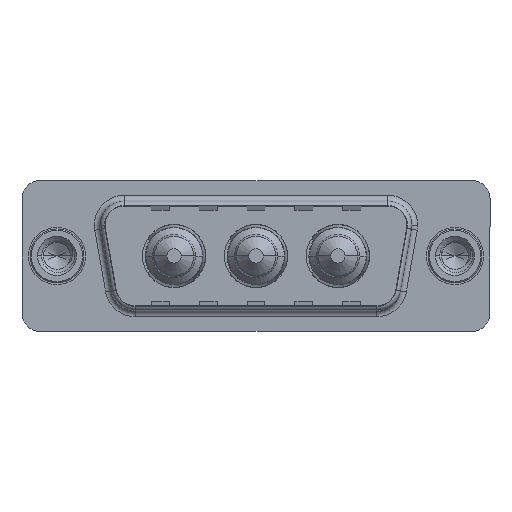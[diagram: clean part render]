
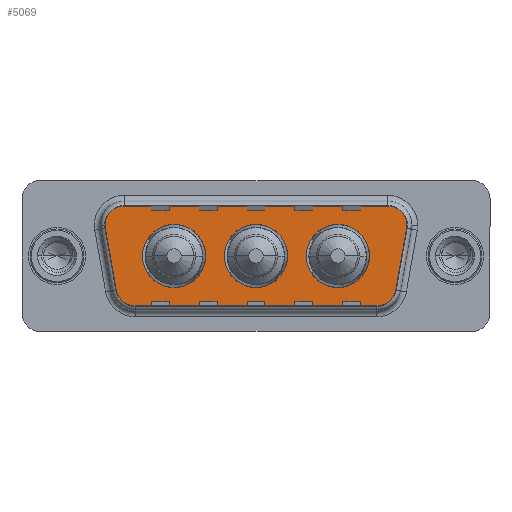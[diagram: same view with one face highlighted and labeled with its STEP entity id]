
A CAD part, top view. The second image highlights one B-rep face of the part: STEP entity #5069.
In plain terms, the highlighted planar face has unit normal (0, 0, 1).
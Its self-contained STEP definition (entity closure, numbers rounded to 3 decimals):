
#84 = VECTOR ( 'NONE', #6820, 1000. ) ;
#132 = EDGE_CURVE ( 'NONE', #2947, #4873, #10648, .T. ) ;
#138 = AXIS2_PLACEMENT_3D ( 'NONE', #4179, #12192, #12235 ) ;
#210 = FACE_OUTER_BOUND ( 'NONE', #10993, .T. ) ;
#246 = CIRCLE ( 'NONE', #1196, 2.65 ) ;
#299 = LINE ( 'NONE', #9183, #2934 ) ;
#313 = EDGE_CURVE ( 'NONE', #2612, #9984, #11903, .T. ) ;
#733 = CARTESIAN_POINT ( 'NONE',  ( 9.8, 0., 0. ) ) ;
#816 = CARTESIAN_POINT ( 'NONE',  ( 19.3, 0., 0. ) ) ;
#866 = ORIENTED_EDGE ( 'NONE', *, *, #8293, .T. ) ;
#870 = VERTEX_POINT ( 'NONE', #6305 ) ;
#885 = CARTESIAN_POINT ( 'NONE',  ( 4.464, -3.247, 0. ) ) ;
#931 = CARTESIAN_POINT ( 'NONE',  ( 29.859, 2.553, 0. ) ) ;
#1159 = AXIS2_PLACEMENT_3D ( 'NONE', #8033, #1216, #9176 ) ;
#1181 = CARTESIAN_POINT ( 'NONE',  ( 6.434, -4.9, 0. ) ) ;
#1196 = AXIS2_PLACEMENT_3D ( 'NONE', #1522, #9487, #2648 ) ;
#1216 = DIRECTION ( 'NONE',  ( 0., 0., 1. ) ) ;
#1222 = DIRECTION ( 'NONE',  ( 0.174, -0.985, 0. ) ) ;
#1249 = EDGE_CURVE ( 'NONE', #8948, #6044, #7623, .T. ) ;
#1389 = CIRCLE ( 'NONE', #4182, 2. ) ;
#1522 = CARTESIAN_POINT ( 'NONE',  ( 16.65, 0., 0. ) ) ;
#1660 = DIRECTION ( 'NONE',  ( 0.174, 0.985, 0. ) ) ;
#1740 = CIRCLE ( 'NONE', #14397, 2. ) ;
#2169 = LINE ( 'NONE', #6223, #13575 ) ;
#2174 = DIRECTION ( 'NONE',  ( 0., 0., 1. ) ) ;
#2392 = ORIENTED_EDGE ( 'NONE', *, *, #12347, .T. ) ;
#2534 = VERTEX_POINT ( 'NONE', #3991 ) ;
#2612 = VERTEX_POINT ( 'NONE', #4914 ) ;
#2648 = DIRECTION ( 'NONE',  ( 1., 0., 0. ) ) ;
#2897 = VERTEX_POINT ( 'NONE', #9864 ) ;
#2934 = VECTOR ( 'NONE', #1222, 1000. ) ;
#2947 = VERTEX_POINT ( 'NONE', #11709 ) ;
#2950 = VERTEX_POINT ( 'NONE', #9781 ) ;
#3056 = AXIS2_PLACEMENT_3D ( 'NONE', #11707, #8734, #14767 ) ;
#3088 = LINE ( 'NONE', #7539, #84 ) ;
#3215 = FACE_BOUND ( 'NONE', #10224, .T. ) ;
#3217 = EDGE_LOOP ( 'NONE', ( #8655, #14427 ) ) ;
#3282 = DIRECTION ( 'NONE',  ( 0., 0., 1. ) ) ;
#3383 = AXIS2_PLACEMENT_3D ( 'NONE', #6081, #5894, #13878 ) ;
#3587 = EDGE_CURVE ( 'NONE', #12411, #5707, #8591, .T. ) ;
#3657 = AXIS2_PLACEMENT_3D ( 'NONE', #733, #2174, #4321 ) ;
#3991 = CARTESIAN_POINT ( 'NONE',  ( 3.441, 2.553, 0. ) ) ;
#4034 = CARTESIAN_POINT ( 'NONE',  ( 5.411, 4.9, 0. ) ) ;
#4156 = CARTESIAN_POINT ( 'NONE',  ( 20.85, 0., 0. ) ) ;
#4179 = CARTESIAN_POINT ( 'NONE',  ( 6.434, -2.9, 0. ) ) ;
#4182 = AXIS2_PLACEMENT_3D ( 'NONE', #13046, #6277, #14203 ) ;
#4273 = CARTESIAN_POINT ( 'NONE',  ( 23.5, 0., 0. ) ) ;
#4315 = DIRECTION ( 'NONE',  ( 0., 0., 1. ) ) ;
#4321 = DIRECTION ( 'NONE',  ( 1., 0., 0. ) ) ;
#4364 = DIRECTION ( 'NONE',  ( 1., 0., 0. ) ) ;
#4834 = EDGE_CURVE ( 'NONE', #9984, #2612, #7172, .T. ) ;
#4873 = VERTEX_POINT ( 'NONE', #816 ) ;
#4914 = CARTESIAN_POINT ( 'NONE',  ( 7.15, 0., 0. ) ) ;
#5069 = ADVANCED_FACE ( 'NONE', ( #6271, #12287, #3215, #210 ), #6508, .T. ) ;
#5159 = CIRCLE ( 'NONE', #9671, 2.65 ) ;
#5178 = VERTEX_POINT ( 'NONE', #4034 ) ;
#5265 = CARTESIAN_POINT ( 'NONE',  ( 26.15, 0., 0. ) ) ;
#5707 = VERTEX_POINT ( 'NONE', #4156 ) ;
#5739 = EDGE_CURVE ( 'NONE', #5707, #12411, #5159, .T. ) ;
#5894 = DIRECTION ( 'NONE',  ( 0., 0., 1. ) ) ;
#6044 = VERTEX_POINT ( 'NONE', #1181 ) ;
#6081 = CARTESIAN_POINT ( 'NONE',  ( 26.866, -2.9, 0. ) ) ;
#6198 = CIRCLE ( 'NONE', #9637, 2. ) ;
#6223 = CARTESIAN_POINT ( 'NONE',  ( 29.859, 2.553, 0. ) ) ;
#6271 = FACE_BOUND ( 'NONE', #8634, .T. ) ;
#6277 = DIRECTION ( 'NONE',  ( 0., 0., 1. ) ) ;
#6305 = CARTESIAN_POINT ( 'NONE',  ( 27.889, 4.9, 0. ) ) ;
#6508 = PLANE ( 'NONE',  #3383 ) ;
#6820 = DIRECTION ( 'NONE',  ( -1., 0., 0. ) ) ;
#7026 = CARTESIAN_POINT ( 'NONE',  ( 26.866, -2.9, 0. ) ) ;
#7172 = CIRCLE ( 'NONE', #3657, 2.65 ) ;
#7311 = EDGE_CURVE ( 'NONE', #2950, #12274, #1740, .T. ) ;
#7320 = CARTESIAN_POINT ( 'NONE',  ( 9.8, 0., 0. ) ) ;
#7323 = EDGE_CURVE ( 'NONE', #2897, #870, #1389, .T. ) ;
#7368 = CARTESIAN_POINT ( 'NONE',  ( 23.5, 0., 0. ) ) ;
#7532 = VERTEX_POINT ( 'NONE', #931 ) ;
#7539 = CARTESIAN_POINT ( 'NONE',  ( 5.411, 4.9, 0. ) ) ;
#7588 = ORIENTED_EDGE ( 'NONE', *, *, #14042, .T. ) ;
#7623 = CIRCLE ( 'NONE', #138, 2. ) ;
#7855 = DIRECTION ( 'NONE',  ( 0., 0., 1. ) ) ;
#8033 = CARTESIAN_POINT ( 'NONE',  ( 27.889, 2.9, 0. ) ) ;
#8293 = EDGE_CURVE ( 'NONE', #5178, #2534, #6198, .T. ) ;
#8394 = CARTESIAN_POINT ( 'NONE',  ( 6.434, -4.9, 0. ) ) ;
#8496 = ORIENTED_EDGE ( 'NONE', *, *, #12301, .T. ) ;
#8591 = CIRCLE ( 'NONE', #14245, 2.65 ) ;
#8634 = EDGE_LOOP ( 'NONE', ( #11627, #13850 ) ) ;
#8655 = ORIENTED_EDGE ( 'NONE', *, *, #3587, .F. ) ;
#8734 = DIRECTION ( 'NONE',  ( 0., 0., 1. ) ) ;
#8948 = VERTEX_POINT ( 'NONE', #885 ) ;
#9142 = EDGE_CURVE ( 'NONE', #2534, #8948, #299, .T. ) ;
#9176 = DIRECTION ( 'NONE',  ( -1., 0., 0. ) ) ;
#9183 = CARTESIAN_POINT ( 'NONE',  ( 3.441, 2.553, 0. ) ) ;
#9192 = ORIENTED_EDGE ( 'NONE', *, *, #9142, .T. ) ;
#9487 = DIRECTION ( 'NONE',  ( 0., 0., 1. ) ) ;
#9509 = ORIENTED_EDGE ( 'NONE', *, *, #11396, .T. ) ;
#9532 = DIRECTION ( 'NONE',  ( 1., 0., 0. ) ) ;
#9637 = AXIS2_PLACEMENT_3D ( 'NONE', #10101, #3282, #11246 ) ;
#9665 = CARTESIAN_POINT ( 'NONE',  ( 12.45, 0., 0. ) ) ;
#9671 = AXIS2_PLACEMENT_3D ( 'NONE', #7368, #10488, #10470 ) ;
#9781 = CARTESIAN_POINT ( 'NONE',  ( 26.866, -4.9, 0. ) ) ;
#9864 = CARTESIAN_POINT ( 'NONE',  ( 29.889, 2.9, 0. ) ) ;
#9984 = VERTEX_POINT ( 'NONE', #9665 ) ;
#10101 = CARTESIAN_POINT ( 'NONE',  ( 5.411, 2.9, 0. ) ) ;
#10224 = EDGE_LOOP ( 'NONE', ( #11722, #13334 ) ) ;
#10470 = DIRECTION ( 'NONE',  ( 1., 0., 0. ) ) ;
#10488 = DIRECTION ( 'NONE',  ( 0., 0., 1. ) ) ;
#10498 = CIRCLE ( 'NONE', #1159, 2. ) ;
#10648 = CIRCLE ( 'NONE', #3056, 2.65 ) ;
#10753 = DIRECTION ( 'NONE',  ( 1., 0., 0. ) ) ;
#10993 = EDGE_LOOP ( 'NONE', ( #11226, #2392, #7588, #11799, #9509, #866, #9192, #14488, #8496 ) ) ;
#11226 = ORIENTED_EDGE ( 'NONE', *, *, #7311, .T. ) ;
#11246 = DIRECTION ( 'NONE',  ( 1., 0., 0. ) ) ;
#11396 = EDGE_CURVE ( 'NONE', #870, #5178, #3088, .T. ) ;
#11618 = LINE ( 'NONE', #8394, #14292 ) ;
#11627 = ORIENTED_EDGE ( 'NONE', *, *, #12267, .F. ) ;
#11707 = CARTESIAN_POINT ( 'NONE',  ( 16.65, 0., 0. ) ) ;
#11709 = CARTESIAN_POINT ( 'NONE',  ( 14., 0., 0. ) ) ;
#11722 = ORIENTED_EDGE ( 'NONE', *, *, #4834, .F. ) ;
#11728 = CARTESIAN_POINT ( 'NONE',  ( 28.836, -3.247, 0. ) ) ;
#11799 = ORIENTED_EDGE ( 'NONE', *, *, #7323, .T. ) ;
#11903 = CIRCLE ( 'NONE', #14519, 2.65 ) ;
#12192 = DIRECTION ( 'NONE',  ( 0., 0., 1. ) ) ;
#12235 = DIRECTION ( 'NONE',  ( -1., 0., 0. ) ) ;
#12267 = EDGE_CURVE ( 'NONE', #4873, #2947, #246, .T. ) ;
#12274 = VERTEX_POINT ( 'NONE', #11728 ) ;
#12287 = FACE_BOUND ( 'NONE', #3217, .T. ) ;
#12301 = EDGE_CURVE ( 'NONE', #6044, #2950, #11618, .T. ) ;
#12347 = EDGE_CURVE ( 'NONE', #12274, #7532, #2169, .T. ) ;
#12411 = VERTEX_POINT ( 'NONE', #5265 ) ;
#12993 = DIRECTION ( 'NONE',  ( 1., 0., 0. ) ) ;
#13046 = CARTESIAN_POINT ( 'NONE',  ( 27.889, 2.9, 0. ) ) ;
#13334 = ORIENTED_EDGE ( 'NONE', *, *, #313, .F. ) ;
#13575 = VECTOR ( 'NONE', #1660, 1000. ) ;
#13850 = ORIENTED_EDGE ( 'NONE', *, *, #132, .F. ) ;
#13878 = DIRECTION ( 'NONE',  ( 1., 0., 0. ) ) ;
#14042 = EDGE_CURVE ( 'NONE', #7532, #2897, #10498, .T. ) ;
#14203 = DIRECTION ( 'NONE',  ( -1., 0., 0. ) ) ;
#14245 = AXIS2_PLACEMENT_3D ( 'NONE', #4273, #4315, #4364 ) ;
#14292 = VECTOR ( 'NONE', #9532, 1000. ) ;
#14296 = DIRECTION ( 'NONE',  ( 0., 0., 1. ) ) ;
#14397 = AXIS2_PLACEMENT_3D ( 'NONE', #7026, #14296, #10753 ) ;
#14427 = ORIENTED_EDGE ( 'NONE', *, *, #5739, .F. ) ;
#14488 = ORIENTED_EDGE ( 'NONE', *, *, #1249, .T. ) ;
#14519 = AXIS2_PLACEMENT_3D ( 'NONE', #7320, #7855, #12993 ) ;
#14767 = DIRECTION ( 'NONE',  ( 1., 0., 0. ) ) ;
